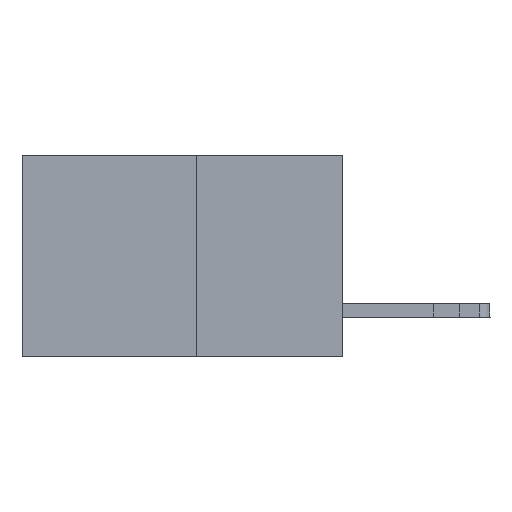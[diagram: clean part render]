
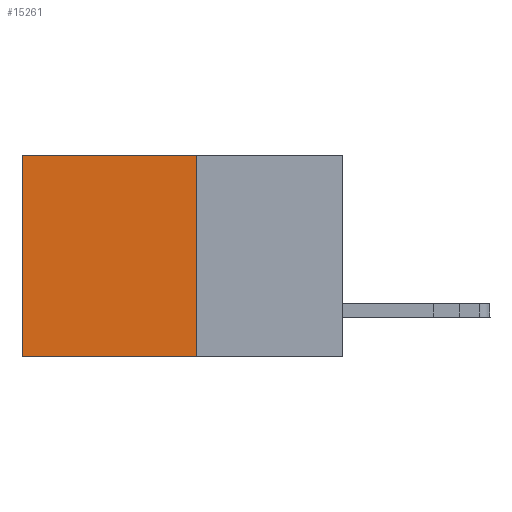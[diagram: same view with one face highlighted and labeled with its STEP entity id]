
A CAD part, left-side view. The second image highlights one B-rep face of the part: STEP entity #15261.
In plain terms, the highlighted planar face has unit normal (-1, 0, 0).
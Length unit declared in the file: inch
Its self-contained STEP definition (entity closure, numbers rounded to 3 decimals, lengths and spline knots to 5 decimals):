
#1005 = CARTESIAN_POINT ( 'NONE',  ( 0.277, 0.27, 0. ) ) ;
#1263 = DIRECTION ( 'NONE',  ( 0., 1., 0. ) ) ;
#1603 = FACE_OUTER_BOUND ( 'NONE', #6092, .T. ) ;
#2108 = VERTEX_POINT ( 'NONE', #9595 ) ;
#2254 = LINE ( 'NONE', #1005, #11680 ) ;
#3737 = VERTEX_POINT ( 'NONE', #5091 ) ;
#4008 = DIRECTION ( 'NONE',  ( 0., 0., -1. ) ) ;
#4786 = CARTESIAN_POINT ( 'NONE',  ( 0.277, 0.59, -0.37 ) ) ;
#5024 = VERTEX_POINT ( 'NONE', #6912 ) ;
#5087 = LINE ( 'NONE', #10326, #12865 ) ;
#5091 = CARTESIAN_POINT ( 'NONE',  ( 0.277, 0.59, -0.37 ) ) ;
#5349 = LINE ( 'NONE', #14091, #10549 ) ;
#5355 = ORIENTED_EDGE ( 'NONE', *, *, #10954, .T. ) ;
#5852 = CARTESIAN_POINT ( 'NONE',  ( 0.277, 0.27, 0. ) ) ;
#6092 = EDGE_LOOP ( 'NONE', ( #5355, #10239, #10953, #15107 ) ) ;
#6676 = DIRECTION ( 'NONE',  ( 1., 0., 0. ) ) ;
#6694 = VECTOR ( 'NONE', #7120, 39.37008 ) ;
#6912 = CARTESIAN_POINT ( 'NONE',  ( 0.277, 0.59, 0. ) ) ;
#7120 = DIRECTION ( 'NONE',  ( 0., 0., -1. ) ) ;
#7671 = EDGE_CURVE ( 'NONE', #13822, #5024, #2254, .T. ) ;
#9420 = CARTESIAN_POINT ( 'NONE',  ( 0.277, 0.27, -0.37 ) ) ;
#9570 = AXIS2_PLACEMENT_3D ( 'NONE', #9420, #6676, #4008 ) ;
#9595 = CARTESIAN_POINT ( 'NONE',  ( 0.277, 0.27, -0.37 ) ) ;
#9761 = EDGE_CURVE ( 'NONE', #2108, #3737, #5087, .T. ) ;
#10239 = ORIENTED_EDGE ( 'NONE', *, *, #9761, .F. ) ;
#10326 = CARTESIAN_POINT ( 'NONE',  ( 0.277, 0.27, -0.37 ) ) ;
#10431 = DIRECTION ( 'NONE',  ( 0., 0., -1. ) ) ;
#10549 = VECTOR ( 'NONE', #10431, 39.37008 ) ;
#10953 = ORIENTED_EDGE ( 'NONE', *, *, #12851, .F. ) ;
#10954 = EDGE_CURVE ( 'NONE', #5024, #3737, #11285, .T. ) ;
#11285 = LINE ( 'NONE', #4786, #6694 ) ;
#11501 = DIRECTION ( 'NONE',  ( 0., 1., 0. ) ) ;
#11680 = VECTOR ( 'NONE', #1263, 39.37008 ) ;
#12851 = EDGE_CURVE ( 'NONE', #13822, #2108, #5349, .T. ) ;
#12865 = VECTOR ( 'NONE', #11501, 39.37008 ) ;
#13822 = VERTEX_POINT ( 'NONE', #5852 ) ;
#14091 = CARTESIAN_POINT ( 'NONE',  ( 0.277, 0.27, -0.37 ) ) ;
#15107 = ORIENTED_EDGE ( 'NONE', *, *, #7671, .T. ) ;
#15261 = ADVANCED_FACE ( 'NONE', ( #1603 ), #15420, .F. ) ;
#15420 = PLANE ( 'NONE',  #9570 ) ;
